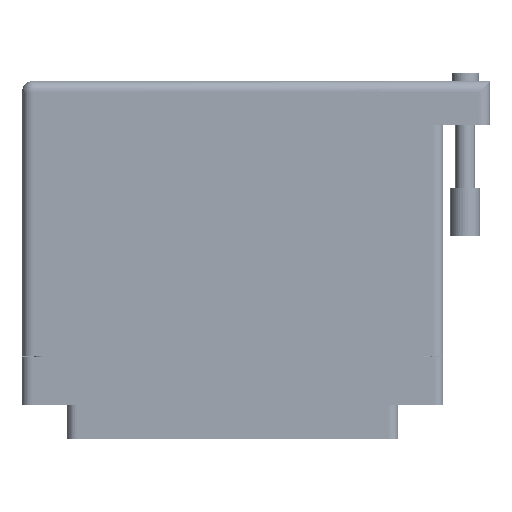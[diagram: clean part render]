
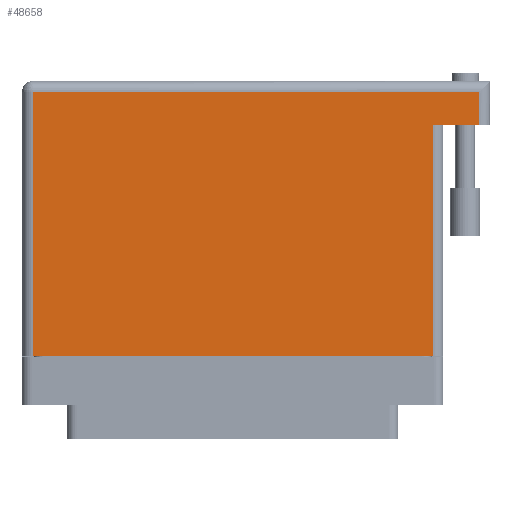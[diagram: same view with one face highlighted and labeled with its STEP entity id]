
A CAD part, front view. The second image highlights one B-rep face of the part: STEP entity #48658.
In plain terms, the highlighted face is planar.
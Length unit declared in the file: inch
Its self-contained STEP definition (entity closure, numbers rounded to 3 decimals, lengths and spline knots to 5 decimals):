
#1132 = EDGE_CURVE ( 'NONE', #51642, #42579, #18590, .T. ) ;
#1453 = DIRECTION ( 'NONE',  ( -1., 0., 0. ) ) ;
#2042 = CARTESIAN_POINT ( 'NONE',  ( 1.589, 1.605, 0.617 ) ) ;
#4446 = CARTESIAN_POINT ( 'NONE',  ( -1.289, -0.1, 0.617 ) ) ;
#6561 = EDGE_CURVE ( 'NONE', #10036, #10411, #60602, .T. ) ;
#8636 = ORIENTED_EDGE ( 'NONE', *, *, #6561, .F. ) ;
#9564 = DIRECTION ( 'NONE',  ( 0., -1., 0. ) ) ;
#9812 = VECTOR ( 'NONE', #1453, 39.37008 ) ;
#10036 = VERTEX_POINT ( 'NONE', #30833 ) ;
#10411 = VERTEX_POINT ( 'NONE', #23055 ) ;
#12314 = VECTOR ( 'NONE', #53223, 39.37008 ) ;
#13227 = VECTOR ( 'NONE', #9564, 39.37008 ) ;
#16727 = AXIS2_PLACEMENT_3D ( 'NONE', #22114, #22861, #39765 ) ;
#18414 = CARTESIAN_POINT ( 'NONE',  ( 1.659, 1.395, 0.617 ) ) ;
#18473 = LINE ( 'NONE', #54015, #72635 ) ;
#18590 = LINE ( 'NONE', #47234, #12314 ) ;
#18861 = FACE_OUTER_BOUND ( 'NONE', #73520, .T. ) ;
#21285 = ORIENTED_EDGE ( 'NONE', *, *, #1132, .T. ) ;
#22114 = CARTESIAN_POINT ( 'NONE',  ( -1.359, 1.675, 0.617 ) ) ;
#22208 = LINE ( 'NONE', #44504, #23959 ) ;
#22861 = DIRECTION ( 'NONE',  ( 0., 0., -1. ) ) ;
#23055 = CARTESIAN_POINT ( 'NONE',  ( 1.289, 1.395, 0.617 ) ) ;
#23959 = VECTOR ( 'NONE', #32911, 39.37008 ) ;
#25823 = LINE ( 'NONE', #38054, #13227 ) ;
#27463 = ORIENTED_EDGE ( 'NONE', *, *, #34521, .T. ) ;
#28557 = ORIENTED_EDGE ( 'NONE', *, *, #38545, .T. ) ;
#28788 = VECTOR ( 'NONE', #47073, 39.37008 ) ;
#30833 = CARTESIAN_POINT ( 'NONE',  ( 1.589, 1.395, 0.617 ) ) ;
#32716 = VERTEX_POINT ( 'NONE', #58040 ) ;
#32911 = DIRECTION ( 'NONE',  ( 0., 1., 0. ) ) ;
#34521 = EDGE_CURVE ( 'NONE', #42579, #10411, #22208, .T. ) ;
#38054 = CARTESIAN_POINT ( 'NONE',  ( -1.289, -0.1, 0.617 ) ) ;
#38545 = EDGE_CURVE ( 'NONE', #10036, #48149, #52792, .T. ) ;
#39765 = DIRECTION ( 'NONE',  ( -1., 0., 0. ) ) ;
#39800 = EDGE_CURVE ( 'NONE', #48149, #32716, #18473, .T. ) ;
#42579 = VERTEX_POINT ( 'NONE', #68110 ) ;
#44504 = CARTESIAN_POINT ( 'NONE',  ( 1.289, 1.395, 0.617 ) ) ;
#45289 = ORIENTED_EDGE ( 'NONE', *, *, #55308, .T. ) ;
#47073 = DIRECTION ( 'NONE',  ( 0., 1., 0. ) ) ;
#47234 = CARTESIAN_POINT ( 'NONE',  ( -1.359, -0.1, 0.617 ) ) ;
#48149 = VERTEX_POINT ( 'NONE', #2042 ) ;
#48658 = ADVANCED_FACE ( 'NONE', ( #18861 ), #51636, .F. ) ;
#51636 = PLANE ( 'NONE',  #16727 ) ;
#51642 = VERTEX_POINT ( 'NONE', #4446 ) ;
#52398 = ORIENTED_EDGE ( 'NONE', *, *, #39800, .T. ) ;
#52792 = LINE ( 'NONE', #58967, #28788 ) ;
#53223 = DIRECTION ( 'NONE',  ( 1., 0., 0. ) ) ;
#54015 = CARTESIAN_POINT ( 'NONE',  ( -1.359, 1.605, 0.617 ) ) ;
#55308 = EDGE_CURVE ( 'NONE', #32716, #51642, #25823, .T. ) ;
#58040 = CARTESIAN_POINT ( 'NONE',  ( -1.289, 1.605, 0.617 ) ) ;
#58967 = CARTESIAN_POINT ( 'NONE',  ( 1.589, 1.675, 0.617 ) ) ;
#59699 = DIRECTION ( 'NONE',  ( -1., 0., 0. ) ) ;
#60602 = LINE ( 'NONE', #18414, #9812 ) ;
#68110 = CARTESIAN_POINT ( 'NONE',  ( 1.289, -0.1, 0.617 ) ) ;
#72635 = VECTOR ( 'NONE', #59699, 39.37008 ) ;
#73520 = EDGE_LOOP ( 'NONE', ( #21285, #27463, #8636, #28557, #52398, #45289 ) ) ;
